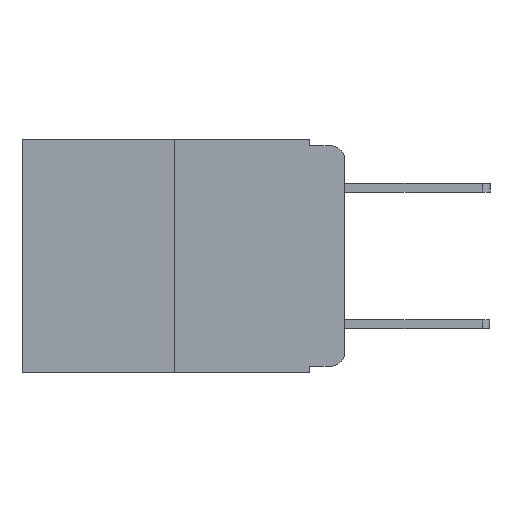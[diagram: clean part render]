
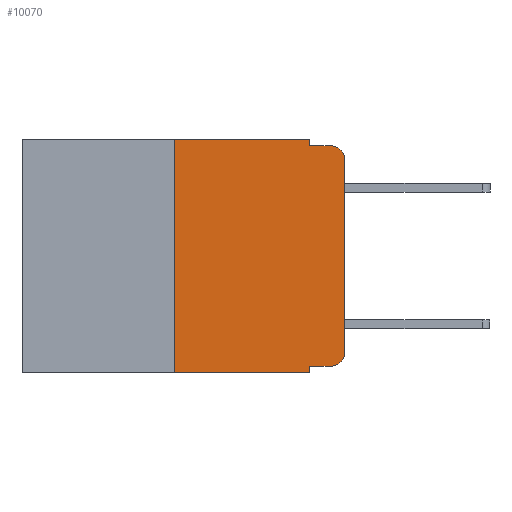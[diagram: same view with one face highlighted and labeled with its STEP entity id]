
A CAD part, left-side view. The second image highlights one B-rep face of the part: STEP entity #10070.
In plain terms, the highlighted planar face has unit normal (-1, 0, 0).
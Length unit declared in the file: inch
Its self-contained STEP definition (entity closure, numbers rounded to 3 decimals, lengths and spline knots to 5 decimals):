
#56 = CARTESIAN_POINT ( 'NONE',  ( 0., 0.051, -0.343 ) ) ;
#466 = CARTESIAN_POINT ( 'NONE',  ( 0., 0.051, 0. ) ) ;
#670 = ORIENTED_EDGE ( 'NONE', *, *, #5816, .F. ) ;
#866 = AXIS2_PLACEMENT_3D ( 'NONE', #2939, #15473, #4784 ) ;
#948 = LINE ( 'NONE', #466, #18858 ) ;
#986 = VECTOR ( 'NONE', #21369, 39.37008 ) ;
#1224 = EDGE_CURVE ( 'NONE', #5241, #22086, #19601, .T. ) ;
#1695 = EDGE_CURVE ( 'NONE', #17831, #16262, #15521, .T. ) ;
#1871 = DIRECTION ( 'NONE',  ( 1., 0., 0. ) ) ;
#1890 = CARTESIAN_POINT ( 'NONE',  ( 0., 0.25, -0.343 ) ) ;
#2868 = CARTESIAN_POINT ( 'NONE',  ( 0., 0.25, 0. ) ) ;
#2939 = CARTESIAN_POINT ( 'NONE',  ( 0., 0.02, -0.313 ) ) ;
#3038 = ORIENTED_EDGE ( 'NONE', *, *, #1224, .F. ) ;
#3703 = EDGE_CURVE ( 'NONE', #5139, #22086, #20873, .T. ) ;
#4172 = CARTESIAN_POINT ( 'NONE',  ( 0., 0., -0.03 ) ) ;
#4630 = EDGE_CURVE ( 'NONE', #11564, #7878, #13763, .T. ) ;
#4784 = DIRECTION ( 'NONE',  ( 0., 0., -1. ) ) ;
#4938 = EDGE_CURVE ( 'NONE', #15366, #5139, #5851, .T. ) ;
#5015 = ORIENTED_EDGE ( 'NONE', *, *, #12451, .F. ) ;
#5139 = VERTEX_POINT ( 'NONE', #4172 ) ;
#5241 = VERTEX_POINT ( 'NONE', #11660 ) ;
#5274 = LINE ( 'NONE', #17346, #14255 ) ;
#5465 = VECTOR ( 'NONE', #13045, 39.37008 ) ;
#5771 = CARTESIAN_POINT ( 'NONE',  ( 0., 0.02, -0.03 ) ) ;
#5783 = FACE_OUTER_BOUND ( 'NONE', #20249, .T. ) ;
#5816 = EDGE_CURVE ( 'NONE', #11564, #10139, #948, .T. ) ;
#5851 = LINE ( 'NONE', #9062, #986 ) ;
#6128 = ORIENTED_EDGE ( 'NONE', *, *, #15009, .T. ) ;
#6797 = DIRECTION ( 'NONE',  ( 0., 0., -1. ) ) ;
#6875 = DIRECTION ( 'NONE',  ( 0., 0., 1. ) ) ;
#7072 = VECTOR ( 'NONE', #19536, 39.37008 ) ;
#7287 = CARTESIAN_POINT ( 'NONE',  ( 0., 0.473, 0. ) ) ;
#7878 = VERTEX_POINT ( 'NONE', #21885 ) ;
#7907 = CARTESIAN_POINT ( 'NONE',  ( 0., 0.051, -0.333 ) ) ;
#8128 = ORIENTED_EDGE ( 'NONE', *, *, #1695, .F. ) ;
#8743 = AXIS2_PLACEMENT_3D ( 'NONE', #5771, #13612, #6797 ) ;
#9062 = CARTESIAN_POINT ( 'NONE',  ( 0., 0., 0. ) ) ;
#9196 = CIRCLE ( 'NONE', #866, 0.02 ) ;
#9732 = DIRECTION ( 'NONE',  ( 0., -1., 0. ) ) ;
#9930 = EDGE_CURVE ( 'NONE', #7878, #15366, #9196, .T. ) ;
#10070 = ADVANCED_FACE ( 'NONE', ( #5783 ), #17889, .F. ) ;
#10139 = VERTEX_POINT ( 'NONE', #56 ) ;
#11143 = CARTESIAN_POINT ( 'NONE',  ( 0., 0.25, 0. ) ) ;
#11564 = VERTEX_POINT ( 'NONE', #15332 ) ;
#11660 = CARTESIAN_POINT ( 'NONE',  ( 0., 0.051, -0.01 ) ) ;
#12451 = EDGE_CURVE ( 'NONE', #16262, #12564, #16534, .T. ) ;
#12536 = CARTESIAN_POINT ( 'NONE',  ( 0., 0.051, -0.01 ) ) ;
#12564 = VERTEX_POINT ( 'NONE', #17946 ) ;
#12602 = ORIENTED_EDGE ( 'NONE', *, *, #3703, .T. ) ;
#12915 = ORIENTED_EDGE ( 'NONE', *, *, #9930, .T. ) ;
#13035 = LINE ( 'NONE', #22797, #17110 ) ;
#13045 = DIRECTION ( 'NONE',  ( 0., -1., 0. ) ) ;
#13191 = DIRECTION ( 'NONE',  ( 0., 0., -1. ) ) ;
#13612 = DIRECTION ( 'NONE',  ( -1., 0., 0. ) ) ;
#13721 = ORIENTED_EDGE ( 'NONE', *, *, #4938, .T. ) ;
#13763 = LINE ( 'NONE', #7907, #17286 ) ;
#14134 = DIRECTION ( 'NONE',  ( 0., 0., -1. ) ) ;
#14255 = VECTOR ( 'NONE', #19098, 39.37008 ) ;
#14348 = CARTESIAN_POINT ( 'NONE',  ( 0., 0.02, -0.01 ) ) ;
#14472 = DIRECTION ( 'NONE',  ( 0., 0., -1. ) ) ;
#15009 = EDGE_CURVE ( 'NONE', #17831, #10139, #5274, .T. ) ;
#15332 = CARTESIAN_POINT ( 'NONE',  ( 0., 0.051, -0.333 ) ) ;
#15345 = ORIENTED_EDGE ( 'NONE', *, *, #21972, .F. ) ;
#15365 = AXIS2_PLACEMENT_3D ( 'NONE', #7287, #1871, #14472 ) ;
#15366 = VERTEX_POINT ( 'NONE', #16572 ) ;
#15473 = DIRECTION ( 'NONE',  ( -1., 0., 0. ) ) ;
#15521 = LINE ( 'NONE', #11143, #20137 ) ;
#16262 = VERTEX_POINT ( 'NONE', #2868 ) ;
#16534 = LINE ( 'NONE', #17794, #7072 ) ;
#16572 = CARTESIAN_POINT ( 'NONE',  ( 0., 0., -0.313 ) ) ;
#17110 = VECTOR ( 'NONE', #14134, 39.37008 ) ;
#17286 = VECTOR ( 'NONE', #9732, 39.37008 ) ;
#17346 = CARTESIAN_POINT ( 'NONE',  ( 0., 0.473, -0.343 ) ) ;
#17794 = CARTESIAN_POINT ( 'NONE',  ( 0., 0.473, 0. ) ) ;
#17831 = VERTEX_POINT ( 'NONE', #1890 ) ;
#17889 = PLANE ( 'NONE',  #15365 ) ;
#17946 = CARTESIAN_POINT ( 'NONE',  ( 0., 0.051, 0. ) ) ;
#18858 = VECTOR ( 'NONE', #13191, 39.37008 ) ;
#19098 = DIRECTION ( 'NONE',  ( 0., -1., 0. ) ) ;
#19536 = DIRECTION ( 'NONE',  ( 0., -1., 0. ) ) ;
#19601 = LINE ( 'NONE', #12536, #5465 ) ;
#19716 = ORIENTED_EDGE ( 'NONE', *, *, #4630, .T. ) ;
#20137 = VECTOR ( 'NONE', #6875, 39.37008 ) ;
#20249 = EDGE_LOOP ( 'NONE', ( #13721, #12602, #3038, #15345, #5015, #8128, #6128, #670, #19716, #12915 ) ) ;
#20873 = CIRCLE ( 'NONE', #8743, 0.02 ) ;
#21369 = DIRECTION ( 'NONE',  ( 0., 0., 1. ) ) ;
#21885 = CARTESIAN_POINT ( 'NONE',  ( 0., 0.02, -0.333 ) ) ;
#21972 = EDGE_CURVE ( 'NONE', #12564, #5241, #13035, .T. ) ;
#22086 = VERTEX_POINT ( 'NONE', #14348 ) ;
#22797 = CARTESIAN_POINT ( 'NONE',  ( 0., 0.051, 0. ) ) ;
